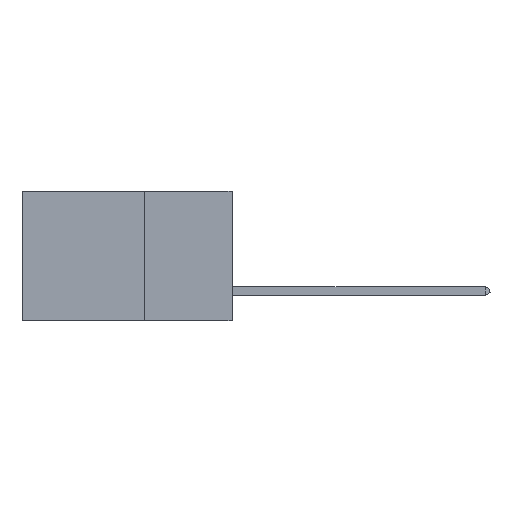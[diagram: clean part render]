
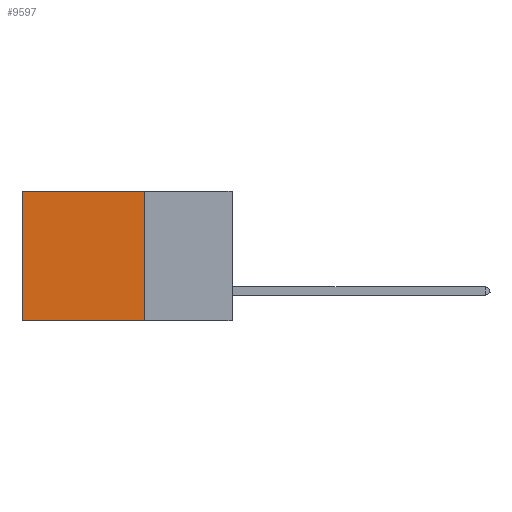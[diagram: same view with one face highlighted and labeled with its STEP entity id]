
A CAD part, left-side view. The second image highlights one B-rep face of the part: STEP entity #9597.
In plain terms, the highlighted planar face has unit normal (-1, 0, 0).
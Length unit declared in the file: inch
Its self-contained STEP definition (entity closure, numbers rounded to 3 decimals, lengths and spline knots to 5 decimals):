
#27 = EDGE_LOOP ( 'NONE', ( #13319, #14180, #2125, #8072 ) ) ;
#602 = EDGE_CURVE ( 'NONE', #2108, #12940, #5047, .T. ) ;
#705 = DIRECTION ( 'NONE',  ( 0., 1., 0. ) ) ;
#1186 = CARTESIAN_POINT ( 'NONE',  ( 0.2875, 0.25, -0.37 ) ) ;
#2108 = VERTEX_POINT ( 'NONE', #7962 ) ;
#2125 = ORIENTED_EDGE ( 'NONE', *, *, #602, .F. ) ;
#2635 = EDGE_CURVE ( 'NONE', #15540, #13156, #6004, .T. ) ;
#4538 = CARTESIAN_POINT ( 'NONE',  ( 0.2875, 0.25, 0. ) ) ;
#4605 = DIRECTION ( 'NONE',  ( 0., 0., -1. ) ) ;
#5047 = LINE ( 'NONE', #12125, #13295 ) ;
#5073 = CARTESIAN_POINT ( 'NONE',  ( 0.2875, 0.6, 0. ) ) ;
#5696 = LINE ( 'NONE', #16987, #8684 ) ;
#6004 = LINE ( 'NONE', #6013, #8541 ) ;
#6013 = CARTESIAN_POINT ( 'NONE',  ( 0.2875, 0.6, 0. ) ) ;
#7311 = DIRECTION ( 'NONE',  ( 1., 0., 0. ) ) ;
#7523 = EDGE_CURVE ( 'NONE', #12940, #13156, #18572, .T. ) ;
#7962 = CARTESIAN_POINT ( 'NONE',  ( 0.2875, 0.25, 0. ) ) ;
#8072 = ORIENTED_EDGE ( 'NONE', *, *, #12248, .T. ) ;
#8541 = VECTOR ( 'NONE', #16775, 39.37008 ) ;
#8560 = AXIS2_PLACEMENT_3D ( 'NONE', #4538, #7311, #4605 ) ;
#8684 = VECTOR ( 'NONE', #705, 39.37008 ) ;
#9597 = ADVANCED_FACE ( 'NONE', ( #18061 ), #11735, .F. ) ;
#11571 = DIRECTION ( 'NONE',  ( 0., 1., 0. ) ) ;
#11735 = PLANE ( 'NONE',  #8560 ) ;
#12125 = CARTESIAN_POINT ( 'NONE',  ( 0.2875, 0.25, 0. ) ) ;
#12248 = EDGE_CURVE ( 'NONE', #2108, #15540, #5696, .T. ) ;
#12940 = VERTEX_POINT ( 'NONE', #14215 ) ;
#13156 = VERTEX_POINT ( 'NONE', #16102 ) ;
#13295 = VECTOR ( 'NONE', #18098, 39.37008 ) ;
#13319 = ORIENTED_EDGE ( 'NONE', *, *, #2635, .T. ) ;
#14180 = ORIENTED_EDGE ( 'NONE', *, *, #7523, .F. ) ;
#14215 = CARTESIAN_POINT ( 'NONE',  ( 0.2875, 0.25, -0.37 ) ) ;
#15540 = VERTEX_POINT ( 'NONE', #5073 ) ;
#16102 = CARTESIAN_POINT ( 'NONE',  ( 0.2875, 0.6, -0.37 ) ) ;
#16472 = VECTOR ( 'NONE', #11571, 39.37008 ) ;
#16775 = DIRECTION ( 'NONE',  ( 0., 0., -1. ) ) ;
#16987 = CARTESIAN_POINT ( 'NONE',  ( 0.2875, 0.25, 0. ) ) ;
#18061 = FACE_OUTER_BOUND ( 'NONE', #27, .T. ) ;
#18098 = DIRECTION ( 'NONE',  ( 0., 0., -1. ) ) ;
#18572 = LINE ( 'NONE', #1186, #16472 ) ;
